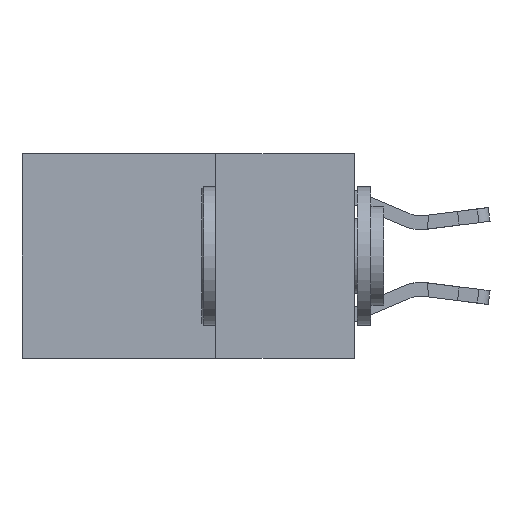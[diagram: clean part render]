
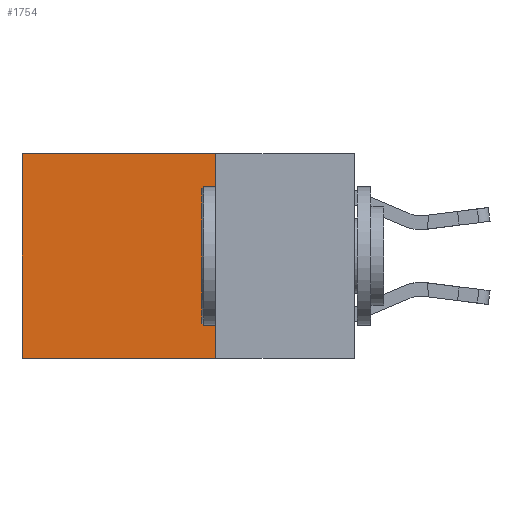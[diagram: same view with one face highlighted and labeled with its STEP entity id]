
A CAD part, left-side view. The second image highlights one B-rep face of the part: STEP entity #1754.
In plain terms, the highlighted planar face has unit normal (-1, 0, 0).
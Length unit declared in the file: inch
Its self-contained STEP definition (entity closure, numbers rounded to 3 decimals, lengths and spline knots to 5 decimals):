
#181 = CARTESIAN_POINT ( 'NONE',  ( 0.2625, 0.25, 0. ) ) ;
#209 = DIRECTION ( 'NONE',  ( 0., 0., -1. ) ) ;
#269 = VECTOR ( 'NONE', #8848, 39.37008 ) ;
#311 = VECTOR ( 'NONE', #9825, 39.37008 ) ;
#662 = CARTESIAN_POINT ( 'NONE',  ( 0.2625, 0.25, -0.37 ) ) ;
#1518 = LINE ( 'NONE', #14866, #269 ) ;
#1754 = ADVANCED_FACE ( 'NONE', ( #3747 ), #12261, .F. ) ;
#2290 = EDGE_CURVE ( 'NONE', #9228, #2433, #6454, .T. ) ;
#2433 = VERTEX_POINT ( 'NONE', #662 ) ;
#2688 = DIRECTION ( 'NONE',  ( 1., 0., 0. ) ) ;
#2726 = LINE ( 'NONE', #4827, #311 ) ;
#2955 = ORIENTED_EDGE ( 'NONE', *, *, #5822, .T. ) ;
#3736 = ORIENTED_EDGE ( 'NONE', *, *, #2290, .F. ) ;
#3747 = FACE_OUTER_BOUND ( 'NONE', #9747, .T. ) ;
#4827 = CARTESIAN_POINT ( 'NONE',  ( 0.2625, 0.6, 0. ) ) ;
#5322 = CARTESIAN_POINT ( 'NONE',  ( 0.2625, 0.25, 0. ) ) ;
#5822 = EDGE_CURVE ( 'NONE', #9228, #9810, #8864, .T. ) ;
#6454 = LINE ( 'NONE', #5322, #14972 ) ;
#6797 = ORIENTED_EDGE ( 'NONE', *, *, #12170, .F. ) ;
#7707 = CARTESIAN_POINT ( 'NONE',  ( 0.2625, 0.6, 0. ) ) ;
#8322 = ORIENTED_EDGE ( 'NONE', *, *, #15500, .T. ) ;
#8848 = DIRECTION ( 'NONE',  ( 0., 1., 0. ) ) ;
#8864 = LINE ( 'NONE', #181, #9091 ) ;
#9091 = VECTOR ( 'NONE', #9979, 39.37008 ) ;
#9118 = DIRECTION ( 'NONE',  ( 0., 0., -1. ) ) ;
#9228 = VERTEX_POINT ( 'NONE', #11568 ) ;
#9747 = EDGE_LOOP ( 'NONE', ( #8322, #6797, #3736, #2955 ) ) ;
#9810 = VERTEX_POINT ( 'NONE', #7707 ) ;
#9825 = DIRECTION ( 'NONE',  ( 0., 0., -1. ) ) ;
#9855 = AXIS2_PLACEMENT_3D ( 'NONE', #11033, #2688, #209 ) ;
#9979 = DIRECTION ( 'NONE',  ( 0., 1., 0. ) ) ;
#10489 = VERTEX_POINT ( 'NONE', #14887 ) ;
#11033 = CARTESIAN_POINT ( 'NONE',  ( 0.2625, 0.25, 0. ) ) ;
#11568 = CARTESIAN_POINT ( 'NONE',  ( 0.2625, 0.25, 0. ) ) ;
#12170 = EDGE_CURVE ( 'NONE', #2433, #10489, #1518, .T. ) ;
#12261 = PLANE ( 'NONE',  #9855 ) ;
#14866 = CARTESIAN_POINT ( 'NONE',  ( 0.2625, 0.25, -0.37 ) ) ;
#14887 = CARTESIAN_POINT ( 'NONE',  ( 0.2625, 0.6, -0.37 ) ) ;
#14972 = VECTOR ( 'NONE', #9118, 39.37008 ) ;
#15500 = EDGE_CURVE ( 'NONE', #9810, #10489, #2726, .T. ) ;
